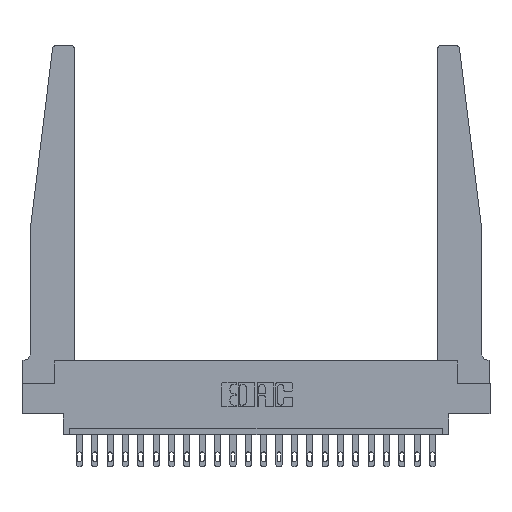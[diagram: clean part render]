
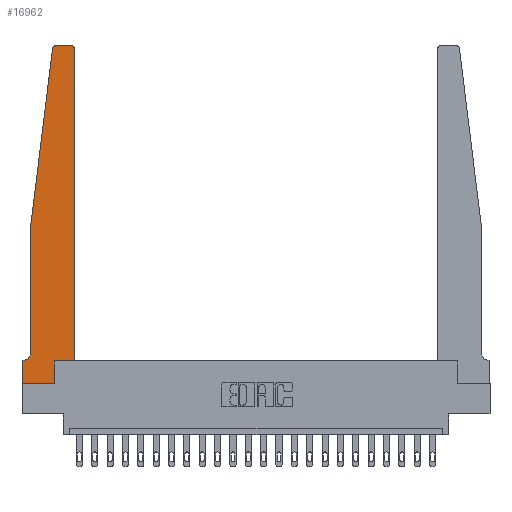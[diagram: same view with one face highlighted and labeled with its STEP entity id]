
A CAD part, top view. The second image highlights one B-rep face of the part: STEP entity #16962.
In plain terms, the highlighted planar face has unit normal (0, 0, 1).
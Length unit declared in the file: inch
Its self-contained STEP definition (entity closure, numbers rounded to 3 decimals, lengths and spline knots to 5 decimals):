
#67 = LINE ( 'NONE', #16146, #618 ) ;
#449 = CARTESIAN_POINT ( 'NONE',  ( 0.2605, 0., 0.37 ) ) ;
#618 = VECTOR ( 'NONE', #12715, 39.37008 ) ;
#715 = VERTEX_POINT ( 'NONE', #449 ) ;
#899 = VERTEX_POINT ( 'NONE', #4386 ) ;
#945 = AXIS2_PLACEMENT_3D ( 'NONE', #8193, #6693, #3386 ) ;
#1022 = CARTESIAN_POINT ( 'NONE',  ( 0., 0., 0.37 ) ) ;
#1157 = CARTESIAN_POINT ( 'NONE',  ( 0.27653, 2.75, 0.37 ) ) ;
#1247 = CARTESIAN_POINT ( 'NONE',  ( 0.425, 0.18, 0.37 ) ) ;
#1264 = VECTOR ( 'NONE', #12537, 39.37008 ) ;
#1488 = DIRECTION ( 'NONE',  ( 1., 0., 0. ) ) ;
#1544 = CARTESIAN_POINT ( 'NONE',  ( 0.24675, 2.72367, 0.37 ) ) ;
#1766 = EDGE_CURVE ( 'NONE', #20719, #20578, #21069, .T. ) ;
#2027 = ORIENTED_EDGE ( 'NONE', *, *, #3603, .T. ) ;
#2039 = AXIS2_PLACEMENT_3D ( 'NONE', #5397, #10880, #16246 ) ;
#2154 = EDGE_CURVE ( 'NONE', #4085, #715, #18421, .T. ) ;
#2527 = VERTEX_POINT ( 'NONE', #11659 ) ;
#2772 = CARTESIAN_POINT ( 'NONE',  ( 0., 0., 0.37 ) ) ;
#2893 = VECTOR ( 'NONE', #18163, 39.37008 ) ;
#3108 = ORIENTED_EDGE ( 'NONE', *, *, #15775, .T. ) ;
#3386 = DIRECTION ( 'NONE',  ( 1., 0., 0. ) ) ;
#3443 = EDGE_CURVE ( 'NONE', #2527, #14660, #10541, .T. ) ;
#3573 = DIRECTION ( 'NONE',  ( -1., 0., 0. ) ) ;
#3603 = EDGE_CURVE ( 'NONE', #4659, #7619, #10056, .T. ) ;
#3978 = CARTESIAN_POINT ( 'NONE',  ( 0.065, 1.25, 0.37 ) ) ;
#4085 = VERTEX_POINT ( 'NONE', #1022 ) ;
#4386 = CARTESIAN_POINT ( 'NONE',  ( 0.425, 2.72, 0.37 ) ) ;
#4572 = DIRECTION ( 'NONE',  ( 0., 0., 1. ) ) ;
#4659 = VERTEX_POINT ( 'NONE', #1544 ) ;
#4677 = CARTESIAN_POINT ( 'NONE',  ( 0.425, 0.18, 0.37 ) ) ;
#4694 = DIRECTION ( 'NONE',  ( -0.122, -0.992, 0. ) ) ;
#5397 = CARTESIAN_POINT ( 'NONE',  ( 0.27653, 2.72, 0.37 ) ) ;
#6048 = DIRECTION ( 'NONE',  ( 0., -1., 0. ) ) ;
#6685 = ORIENTED_EDGE ( 'NONE', *, *, #7785, .T. ) ;
#6693 = DIRECTION ( 'NONE',  ( 0., 0., 1. ) ) ;
#6803 = AXIS2_PLACEMENT_3D ( 'NONE', #21245, #9136, #12342 ) ;
#7121 = CARTESIAN_POINT ( 'NONE',  ( 0.25, 2.75, 0.37 ) ) ;
#7170 = ORIENTED_EDGE ( 'NONE', *, *, #18640, .T. ) ;
#7377 = EDGE_CURVE ( 'NONE', #20578, #4659, #12620, .T. ) ;
#7450 = DIRECTION ( 'NONE',  ( 0., 1., 0. ) ) ;
#7619 = VERTEX_POINT ( 'NONE', #12006 ) ;
#7785 = EDGE_CURVE ( 'NONE', #18263, #2527, #11557, .T. ) ;
#7929 = AXIS2_PLACEMENT_3D ( 'NONE', #22056, #4572, #1488 ) ;
#8193 = CARTESIAN_POINT ( 'NONE',  ( 0., 0.1875, 0.37 ) ) ;
#8292 = CIRCLE ( 'NONE', #7929, 0.03 ) ;
#9136 = DIRECTION ( 'NONE',  ( 0., 0., -1. ) ) ;
#9363 = ORIENTED_EDGE ( 'NONE', *, *, #20601, .T. ) ;
#9432 = ORIENTED_EDGE ( 'NONE', *, *, #2154, .T. ) ;
#9463 = EDGE_CURVE ( 'NONE', #14660, #4085, #21953, .T. ) ;
#10056 = LINE ( 'NONE', #20339, #11046 ) ;
#10541 = LINE ( 'NONE', #19217, #20156 ) ;
#10880 = DIRECTION ( 'NONE',  ( 0., 0., 1. ) ) ;
#11046 = VECTOR ( 'NONE', #4694, 39.37008 ) ;
#11431 = CARTESIAN_POINT ( 'NONE',  ( 0., 0., 0.37 ) ) ;
#11521 = ORIENTED_EDGE ( 'NONE', *, *, #11781, .T. ) ;
#11557 = CIRCLE ( 'NONE', #6803, 0.05 ) ;
#11659 = CARTESIAN_POINT ( 'NONE',  ( 0.015, 0.1875, 0.37 ) ) ;
#11690 = DIRECTION ( 'NONE',  ( 1., 0., 0. ) ) ;
#11736 = FACE_OUTER_BOUND ( 'NONE', #12124, .T. ) ;
#11779 = ORIENTED_EDGE ( 'NONE', *, *, #7377, .T. ) ;
#11781 = EDGE_CURVE ( 'NONE', #715, #16390, #17959, .T. ) ;
#12006 = CARTESIAN_POINT ( 'NONE',  ( 0.065, 1.25, 0.37 ) ) ;
#12124 = EDGE_LOOP ( 'NONE', ( #15393, #11779, #2027, #3108, #6685, #12716, #19740, #9432, #11521, #12986, #7170, #9363 ) ) ;
#12342 = DIRECTION ( 'NONE',  ( -1., 0., 0. ) ) ;
#12433 = VERTEX_POINT ( 'NONE', #4677 ) ;
#12440 = EDGE_CURVE ( 'NONE', #16390, #12433, #21938, .T. ) ;
#12537 = DIRECTION ( 'NONE',  ( 0., -1., 0. ) ) ;
#12620 = CIRCLE ( 'NONE', #2039, 0.03 ) ;
#12715 = DIRECTION ( 'NONE',  ( 0., 1., 0. ) ) ;
#12716 = ORIENTED_EDGE ( 'NONE', *, *, #3443, .T. ) ;
#12986 = ORIENTED_EDGE ( 'NONE', *, *, #12440, .T. ) ;
#13988 = CARTESIAN_POINT ( 'NONE',  ( 0.065, 0.2375, 0.37 ) ) ;
#14315 = VECTOR ( 'NONE', #15816, 39.37008 ) ;
#14660 = VERTEX_POINT ( 'NONE', #18016 ) ;
#15096 = CARTESIAN_POINT ( 'NONE',  ( 0.395, 2.75, 0.37 ) ) ;
#15152 = PLANE ( 'NONE',  #945 ) ;
#15393 = ORIENTED_EDGE ( 'NONE', *, *, #1766, .T. ) ;
#15633 = VECTOR ( 'NONE', #7450, 39.37008 ) ;
#15775 = EDGE_CURVE ( 'NONE', #7619, #18263, #21227, .T. ) ;
#15816 = DIRECTION ( 'NONE',  ( -1., 0., 0. ) ) ;
#16146 = CARTESIAN_POINT ( 'NONE',  ( 0.425, 0.18, 0.37 ) ) ;
#16246 = DIRECTION ( 'NONE',  ( 1., 0., 0. ) ) ;
#16360 = CARTESIAN_POINT ( 'NONE',  ( 0.2605, 0.18, 0.37 ) ) ;
#16390 = VERTEX_POINT ( 'NONE', #20500 ) ;
#16962 = ADVANCED_FACE ( 'NONE', ( #11736 ), #15152, .T. ) ;
#17959 = LINE ( 'NONE', #16360, #15633 ) ;
#18016 = CARTESIAN_POINT ( 'NONE',  ( 0., 0.1875, 0.37 ) ) ;
#18163 = DIRECTION ( 'NONE',  ( 1., 0., 0. ) ) ;
#18263 = VERTEX_POINT ( 'NONE', #13988 ) ;
#18421 = LINE ( 'NONE', #2772, #20174 ) ;
#18640 = EDGE_CURVE ( 'NONE', #12433, #899, #67, .T. ) ;
#19217 = CARTESIAN_POINT ( 'NONE',  ( 0.065, 0.1875, 0.37 ) ) ;
#19740 = ORIENTED_EDGE ( 'NONE', *, *, #9463, .T. ) ;
#20156 = VECTOR ( 'NONE', #3573, 39.37008 ) ;
#20174 = VECTOR ( 'NONE', #11690, 39.37008 ) ;
#20339 = CARTESIAN_POINT ( 'NONE',  ( 0.065, 1.25, 0.37 ) ) ;
#20500 = CARTESIAN_POINT ( 'NONE',  ( 0.2605, 0.18, 0.37 ) ) ;
#20578 = VERTEX_POINT ( 'NONE', #1157 ) ;
#20601 = EDGE_CURVE ( 'NONE', #899, #20719, #8292, .T. ) ;
#20666 = VECTOR ( 'NONE', #6048, 39.37008 ) ;
#20719 = VERTEX_POINT ( 'NONE', #15096 ) ;
#21069 = LINE ( 'NONE', #7121, #14315 ) ;
#21227 = LINE ( 'NONE', #3978, #1264 ) ;
#21245 = CARTESIAN_POINT ( 'NONE',  ( 0.015, 0.2375, 0.37 ) ) ;
#21938 = LINE ( 'NONE', #1247, #2893 ) ;
#21953 = LINE ( 'NONE', #11431, #20666 ) ;
#22056 = CARTESIAN_POINT ( 'NONE',  ( 0.395, 2.72, 0.37 ) ) ;
